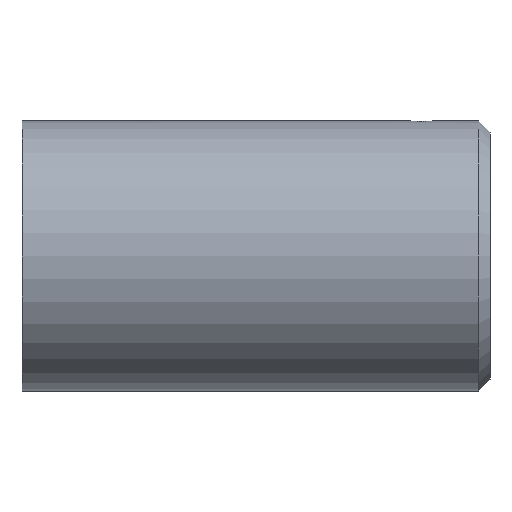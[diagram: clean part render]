
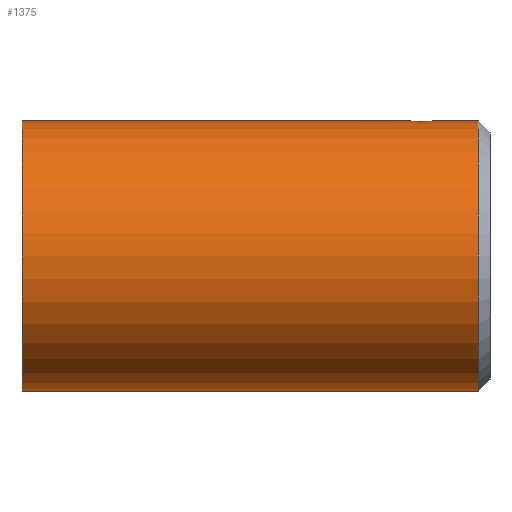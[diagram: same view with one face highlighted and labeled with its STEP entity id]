
A CAD part, front view. The second image highlights one B-rep face of the part: STEP entity #1375.
In plain terms, the highlighted cylindrical face has radius 17.571 mm (diameter 35.142 mm), a full revolution.
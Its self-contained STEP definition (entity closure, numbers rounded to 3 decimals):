
#96=FACE_BOUND('',#229,.T.);
#100=CIRCLE('',#1475,17.571);
#101=CIRCLE('',#1476,17.571);
#143=FACE_OUTER_BOUND('',#228,.T.);
#228=EDGE_LOOP('',(#951,#952,#953,#954));
#229=EDGE_LOOP('',(#955,#956));
#341=B_SPLINE_CURVE_WITH_KNOTS('',3,(#2464,#2465,#2466,#2467,#2468,#2469,
#2470,#2471,#2472,#2473),.UNSPECIFIED.,.F.,.F.,(4,2,2,2,4),(0.678,
0.735,0.791,0.848,0.905),
 .UNSPECIFIED.);
#342=B_SPLINE_CURVE_WITH_KNOTS('',3,(#2474,#2475,#2476,#2477,#2478,#2479,
#2480,#2481,#2482,#2483,#2484,#2485,#2486,#2487,#2488,#2489,#2490,#2491,
#2492,#2493,#2494,#2495,#2496,#2497,#2498,#2499),.UNSPECIFIED.,.F.,.F.,
(4,2,2,2,2,2,2,2,2,2,2,2,4),(0.,0.057,0.113,0.17,
0.226,0.283,0.339,0.396,
0.452,0.509,0.565,0.622,
0.678),.UNSPECIFIED.);
#412=LINE('',#2460,#487);
#487=VECTOR('',#1614,18.071);
#588=VERTEX_POINT('',#2457);
#589=VERTEX_POINT('',#2459);
#590=VERTEX_POINT('',#2462);
#591=VERTEX_POINT('',#2463);
#728=EDGE_CURVE('',#588,#588,#100,.F.);
#729=EDGE_CURVE('',#588,#589,#412,.T.);
#730=EDGE_CURVE('',#589,#589,#101,.F.);
#731=EDGE_CURVE('',#590,#591,#341,.F.);
#732=EDGE_CURVE('',#591,#590,#342,.F.);
#951=ORIENTED_EDGE('',*,*,#728,.F.);
#952=ORIENTED_EDGE('',*,*,#729,.T.);
#953=ORIENTED_EDGE('',*,*,#730,.F.);
#954=ORIENTED_EDGE('',*,*,#729,.F.);
#955=ORIENTED_EDGE('',*,*,#731,.T.);
#956=ORIENTED_EDGE('',*,*,#732,.T.);
#1358=CYLINDRICAL_SURFACE('',#1474,17.571);
#1375=ADVANCED_FACE('',(#143,#96),#1358,.T.);
#1474=AXIS2_PLACEMENT_3D('',#2456,#1610,#1611);
#1475=AXIS2_PLACEMENT_3D('',#2458,#1612,#1613);
#1476=AXIS2_PLACEMENT_3D('',#2461,#1615,#1616);
#1610=DIRECTION('center_axis',(1.,0.,0.));
#1611=DIRECTION('ref_axis',(0.,-1.,0.));
#1612=DIRECTION('center_axis',(-1.,0.,0.));
#1613=DIRECTION('ref_axis',(0.,-1.,0.));
#1614=DIRECTION('',(-1.,0.,0.));
#1615=DIRECTION('center_axis',(1.,0.,0.));
#1616=DIRECTION('ref_axis',(0.,-1.,0.));
#2456=CARTESIAN_POINT('Origin',(342.264,184.064,13.948));
#2457=CARTESIAN_POINT('',(392.654,201.635,13.948));
#2458=CARTESIAN_POINT('Origin',(392.654,184.064,13.948));
#2459=CARTESIAN_POINT('',(333.252,201.635,13.948));
#2460=CARTESIAN_POINT('',(342.264,201.635,13.948));
#2461=CARTESIAN_POINT('Origin',(333.252,184.064,13.948));
#2462=CARTESIAN_POINT('',(385.244,182.542,31.453));
#2463=CARTESIAN_POINT('',(383.744,184.042,31.519));
#2464=CARTESIAN_POINT('Ctrl Pts',(383.744,184.042,31.519));
#2465=CARTESIAN_POINT('Ctrl Pts',(383.744,183.853,31.519));
#2466=CARTESIAN_POINT('Ctrl Pts',(383.781,183.652,31.516));
#2467=CARTESIAN_POINT('Ctrl Pts',(383.934,183.283,31.503));
#2468=CARTESIAN_POINT('Ctrl Pts',(384.05,183.114,31.494));
#2469=CARTESIAN_POINT('Ctrl Pts',(384.316,182.848,31.478));
#2470=CARTESIAN_POINT('Ctrl Pts',(384.485,182.733,31.469));
#2471=CARTESIAN_POINT('Ctrl Pts',(384.854,182.58,31.457));
#2472=CARTESIAN_POINT('Ctrl Pts',(385.055,182.542,31.453));
#2473=CARTESIAN_POINT('Ctrl Pts',(385.244,182.542,31.453));
#2474=CARTESIAN_POINT('Ctrl Pts',(385.244,182.542,31.453));
#2475=CARTESIAN_POINT('Ctrl Pts',(385.432,182.542,31.453));
#2476=CARTESIAN_POINT('Ctrl Pts',(385.633,182.58,31.457));
#2477=CARTESIAN_POINT('Ctrl Pts',(386.003,182.733,31.469));
#2478=CARTESIAN_POINT('Ctrl Pts',(386.171,182.848,31.478));
#2479=CARTESIAN_POINT('Ctrl Pts',(386.437,183.114,31.494));
#2480=CARTESIAN_POINT('Ctrl Pts',(386.553,183.283,31.503));
#2481=CARTESIAN_POINT('Ctrl Pts',(386.706,183.652,31.516));
#2482=CARTESIAN_POINT('Ctrl Pts',(386.744,183.853,31.519));
#2483=CARTESIAN_POINT('Ctrl Pts',(386.744,184.23,31.52));
#2484=CARTESIAN_POINT('Ctrl Pts',(386.706,184.431,31.517));
#2485=CARTESIAN_POINT('Ctrl Pts',(386.553,184.801,31.505));
#2486=CARTESIAN_POINT('Ctrl Pts',(386.437,184.969,31.497));
#2487=CARTESIAN_POINT('Ctrl Pts',(386.171,185.236,31.481));
#2488=CARTESIAN_POINT('Ctrl Pts',(386.003,185.351,31.472));
#2489=CARTESIAN_POINT('Ctrl Pts',(385.633,185.504,31.461));
#2490=CARTESIAN_POINT('Ctrl Pts',(385.432,185.542,31.457));
#2491=CARTESIAN_POINT('Ctrl Pts',(385.055,185.542,31.457));
#2492=CARTESIAN_POINT('Ctrl Pts',(384.854,185.504,31.461));
#2493=CARTESIAN_POINT('Ctrl Pts',(384.485,185.351,31.472));
#2494=CARTESIAN_POINT('Ctrl Pts',(384.316,185.236,31.481));
#2495=CARTESIAN_POINT('Ctrl Pts',(384.05,184.969,31.497));
#2496=CARTESIAN_POINT('Ctrl Pts',(383.934,184.801,31.505));
#2497=CARTESIAN_POINT('Ctrl Pts',(383.781,184.431,31.517));
#2498=CARTESIAN_POINT('Ctrl Pts',(383.744,184.23,31.52));
#2499=CARTESIAN_POINT('Ctrl Pts',(383.744,184.042,31.519));
